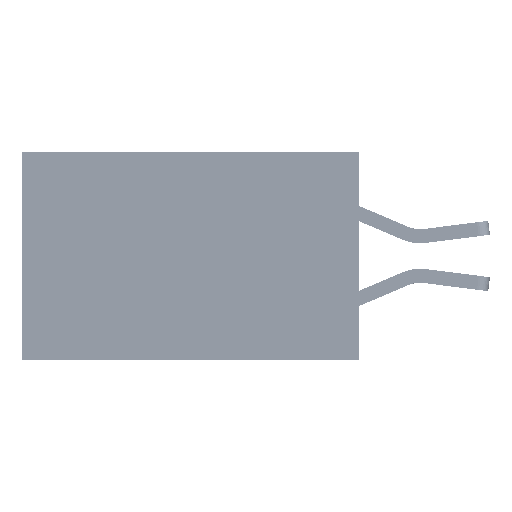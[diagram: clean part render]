
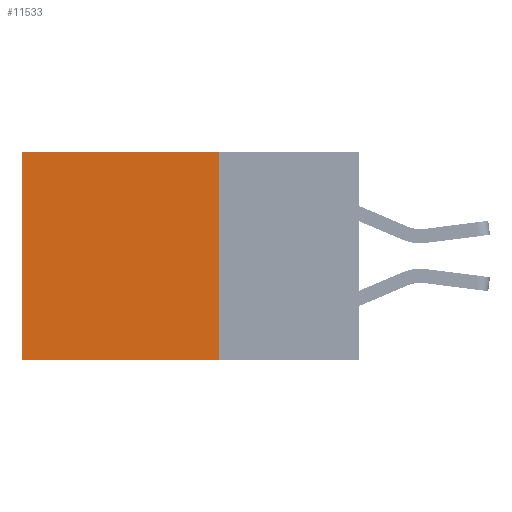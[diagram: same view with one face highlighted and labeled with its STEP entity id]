
A CAD part, left-side view. The second image highlights one B-rep face of the part: STEP entity #11533.
In plain terms, the highlighted planar face has unit normal (-1, 0, 0).
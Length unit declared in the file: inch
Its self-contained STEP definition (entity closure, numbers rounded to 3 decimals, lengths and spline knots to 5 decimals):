
#1570 = PLANE ( 'NONE',  #3063 ) ;
#3063 = AXIS2_PLACEMENT_3D ( 'NONE', #19715, #16365, #28388 ) ;
#3756 = LINE ( 'NONE', #12844, #23546 ) ;
#3829 = VECTOR ( 'NONE', #10021, 39.37008 ) ;
#4122 = ORIENTED_EDGE ( 'NONE', *, *, #29698, .T. ) ;
#10021 = DIRECTION ( 'NONE',  ( 0., 0., -1. ) ) ;
#11533 = ADVANCED_FACE ( 'NONE', ( #16752 ), #1570, .F. ) ;
#11986 = EDGE_CURVE ( 'NONE', #38269, #18502, #34051, .T. ) ;
#12844 = CARTESIAN_POINT ( 'NONE',  ( 0.2875, 0.25, 0. ) ) ;
#15598 = DIRECTION ( 'NONE',  ( 0., 1., 0. ) ) ;
#16130 = CARTESIAN_POINT ( 'NONE',  ( 0.2875, 0.6, 0. ) ) ;
#16365 = DIRECTION ( 'NONE',  ( 1., 0., 0. ) ) ;
#16585 = VERTEX_POINT ( 'NONE', #33455 ) ;
#16752 = FACE_OUTER_BOUND ( 'NONE', #19250, .T. ) ;
#17295 = ORIENTED_EDGE ( 'NONE', *, *, #11986, .F. ) ;
#17411 = DIRECTION ( 'NONE',  ( 0., 0., -1. ) ) ;
#18502 = VERTEX_POINT ( 'NONE', #35322 ) ;
#18964 = ORIENTED_EDGE ( 'NONE', *, *, #30864, .F. ) ;
#19079 = DIRECTION ( 'NONE',  ( 0., 1., 0. ) ) ;
#19250 = EDGE_LOOP ( 'NONE', ( #23423, #17295, #18964, #4122 ) ) ;
#19715 = CARTESIAN_POINT ( 'NONE',  ( 0.2875, 0.25, 0. ) ) ;
#21666 = LINE ( 'NONE', #16130, #3829 ) ;
#21809 = VECTOR ( 'NONE', #17411, 39.37008 ) ;
#23423 = ORIENTED_EDGE ( 'NONE', *, *, #28434, .T. ) ;
#23546 = VECTOR ( 'NONE', #15598, 39.37008 ) ;
#25056 = VECTOR ( 'NONE', #19079, 39.37008 ) ;
#28388 = DIRECTION ( 'NONE',  ( 0., 0., -1. ) ) ;
#28434 = EDGE_CURVE ( 'NONE', #16585, #18502, #21666, .T. ) ;
#29698 = EDGE_CURVE ( 'NONE', #30256, #16585, #3756, .T. ) ;
#30152 = CARTESIAN_POINT ( 'NONE',  ( 0.2875, 0.25, 0. ) ) ;
#30256 = VERTEX_POINT ( 'NONE', #30152 ) ;
#30864 = EDGE_CURVE ( 'NONE', #30256, #38269, #38102, .T. ) ;
#30902 = CARTESIAN_POINT ( 'NONE',  ( 0.2875, 0.25, -0.37 ) ) ;
#33339 = CARTESIAN_POINT ( 'NONE',  ( 0.2875, 0.25, -0.37 ) ) ;
#33455 = CARTESIAN_POINT ( 'NONE',  ( 0.2875, 0.6, 0. ) ) ;
#34051 = LINE ( 'NONE', #30902, #25056 ) ;
#35322 = CARTESIAN_POINT ( 'NONE',  ( 0.2875, 0.6, -0.37 ) ) ;
#38102 = LINE ( 'NONE', #38688, #21809 ) ;
#38269 = VERTEX_POINT ( 'NONE', #33339 ) ;
#38688 = CARTESIAN_POINT ( 'NONE',  ( 0.2875, 0.25, 0. ) ) ;
